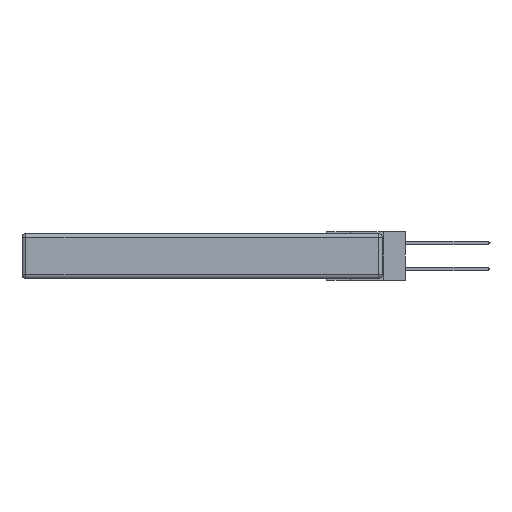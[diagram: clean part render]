
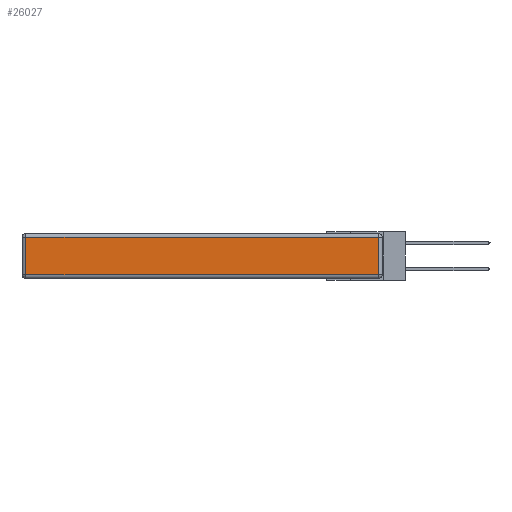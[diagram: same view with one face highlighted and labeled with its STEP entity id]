
A CAD part, left-side view. The second image highlights one B-rep face of the part: STEP entity #26027.
In plain terms, the highlighted planar face has unit normal (-1, 0, 0).
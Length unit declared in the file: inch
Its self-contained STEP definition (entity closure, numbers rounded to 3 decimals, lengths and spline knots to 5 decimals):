
#1110 = CARTESIAN_POINT ( 'NONE',  ( 0., 2.72, -0.343 ) ) ;
#1370 = CARTESIAN_POINT ( 'NONE',  ( 0., 0.03, -0.343 ) ) ;
#1666 = ORIENTED_EDGE ( 'NONE', *, *, #23567, .T. ) ;
#1705 = DIRECTION ( 'NONE',  ( 0., -1., 0. ) ) ;
#2806 = ORIENTED_EDGE ( 'NONE', *, *, #4691, .T. ) ;
#3457 = VECTOR ( 'NONE', #1705, 39.37008 ) ;
#4691 = EDGE_CURVE ( 'NONE', #24152, #14388, #9067, .T. ) ;
#5480 = ORIENTED_EDGE ( 'NONE', *, *, #8796, .T. ) ;
#8796 = EDGE_CURVE ( 'NONE', #20678, #25968, #16475, .T. ) ;
#9067 = LINE ( 'NONE', #23417, #11758 ) ;
#10017 = CARTESIAN_POINT ( 'NONE',  ( 0., 0., -0.343 ) ) ;
#10656 = AXIS2_PLACEMENT_3D ( 'NONE', #10017, #29478, #19462 ) ;
#10739 = EDGE_LOOP ( 'NONE', ( #5480, #30763, #2806, #1666 ) ) ;
#10887 = CARTESIAN_POINT ( 'NONE',  ( 0., 0.03, -0.03 ) ) ;
#11037 = DIRECTION ( 'NONE',  ( 0., 0., -1. ) ) ;
#11349 = VECTOR ( 'NONE', #11037, 39.37008 ) ;
#11758 = VECTOR ( 'NONE', #18230, 39.37008 ) ;
#14388 = VERTEX_POINT ( 'NONE', #31320 ) ;
#16475 = LINE ( 'NONE', #29615, #3457 ) ;
#16743 = CARTESIAN_POINT ( 'NONE',  ( 0., 2.72, -0.313 ) ) ;
#18186 = VECTOR ( 'NONE', #23449, 39.37008 ) ;
#18230 = DIRECTION ( 'NONE',  ( 0., 1., 0. ) ) ;
#19462 = DIRECTION ( 'NONE',  ( 0., 0., 1. ) ) ;
#20678 = VERTEX_POINT ( 'NONE', #16743 ) ;
#21537 = FACE_OUTER_BOUND ( 'NONE', #10739, .T. ) ;
#22098 = PLANE ( 'NONE',  #10656 ) ;
#23102 = LINE ( 'NONE', #1370, #18186 ) ;
#23417 = CARTESIAN_POINT ( 'NONE',  ( 0., 2.75, -0.03 ) ) ;
#23449 = DIRECTION ( 'NONE',  ( 0., 0., 1. ) ) ;
#23567 = EDGE_CURVE ( 'NONE', #14388, #20678, #26615, .T. ) ;
#24151 = EDGE_CURVE ( 'NONE', #25968, #24152, #23102, .T. ) ;
#24152 = VERTEX_POINT ( 'NONE', #10887 ) ;
#25968 = VERTEX_POINT ( 'NONE', #28641 ) ;
#26027 = ADVANCED_FACE ( 'NONE', ( #21537 ), #22098, .T. ) ;
#26615 = LINE ( 'NONE', #1110, #11349 ) ;
#28641 = CARTESIAN_POINT ( 'NONE',  ( 0., 0.03, -0.313 ) ) ;
#29478 = DIRECTION ( 'NONE',  ( -1., 0., 0. ) ) ;
#29615 = CARTESIAN_POINT ( 'NONE',  ( 0., 0., -0.313 ) ) ;
#30763 = ORIENTED_EDGE ( 'NONE', *, *, #24151, .T. ) ;
#31320 = CARTESIAN_POINT ( 'NONE',  ( 0., 2.72, -0.03 ) ) ;
